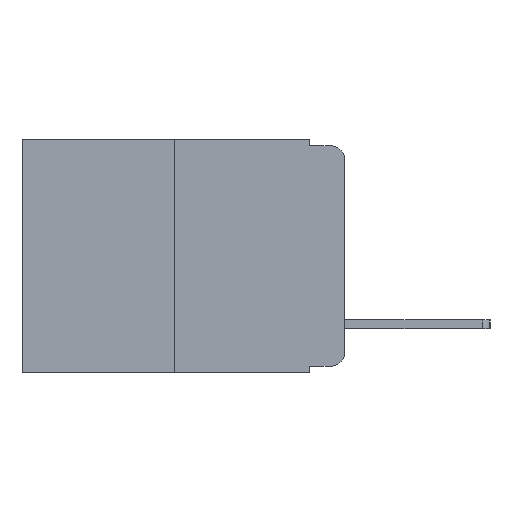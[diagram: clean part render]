
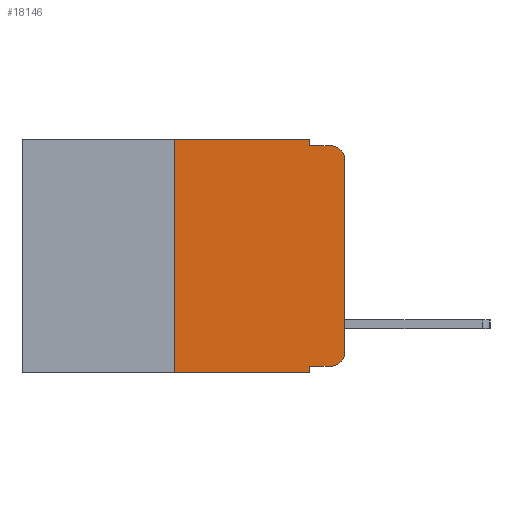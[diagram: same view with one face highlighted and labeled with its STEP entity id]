
A CAD part, left-side view. The second image highlights one B-rep face of the part: STEP entity #18146.
In plain terms, the highlighted planar face has unit normal (-1, 0, 0).
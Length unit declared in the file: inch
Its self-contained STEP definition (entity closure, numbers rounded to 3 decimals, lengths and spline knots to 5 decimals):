
#328 = AXIS2_PLACEMENT_3D ( 'NONE', #8429, #19438, #10042 ) ;
#386 = AXIS2_PLACEMENT_3D ( 'NONE', #10766, #968, #12371 ) ;
#431 = LINE ( 'NONE', #15893, #12927 ) ;
#816 = CIRCLE ( 'NONE', #328, 0.02 ) ;
#943 = EDGE_CURVE ( 'NONE', #11320, #11795, #19920, .T. ) ;
#951 = CARTESIAN_POINT ( 'NONE',  ( 0., 0.02, -0.01 ) ) ;
#968 = DIRECTION ( 'NONE',  ( -1., 0., 0. ) ) ;
#1155 = EDGE_LOOP ( 'NONE', ( #12456, #8713, #17116, #17584, #10220, #2592, #6957, #20031, #3626, #12221 ) ) ;
#1564 = VECTOR ( 'NONE', #10940, 39.37008 ) ;
#2380 = CARTESIAN_POINT ( 'NONE',  ( 0., 0.051, -0.01 ) ) ;
#2413 = VERTEX_POINT ( 'NONE', #951 ) ;
#2592 = ORIENTED_EDGE ( 'NONE', *, *, #20631, .F. ) ;
#2899 = VERTEX_POINT ( 'NONE', #9085 ) ;
#3194 = EDGE_CURVE ( 'NONE', #11320, #19256, #9002, .T. ) ;
#3611 = DIRECTION ( 'NONE',  ( 0., -1., 0. ) ) ;
#3626 = ORIENTED_EDGE ( 'NONE', *, *, #3194, .T. ) ;
#4764 = CARTESIAN_POINT ( 'NONE',  ( 0., 0.051, -0.333 ) ) ;
#4831 = VERTEX_POINT ( 'NONE', #5132 ) ;
#5132 = CARTESIAN_POINT ( 'NONE',  ( 0., 0.051, 0. ) ) ;
#5182 = CARTESIAN_POINT ( 'NONE',  ( 0., 0.02, -0.333 ) ) ;
#5317 = CIRCLE ( 'NONE', #386, 0.02 ) ;
#5368 = PLANE ( 'NONE',  #10641 ) ;
#5703 = VECTOR ( 'NONE', #14656, 39.37008 ) ;
#5969 = LINE ( 'NONE', #15633, #1564 ) ;
#6224 = CARTESIAN_POINT ( 'NONE',  ( 0., 0.051, 0. ) ) ;
#6516 = EDGE_CURVE ( 'NONE', #19256, #17461, #816, .T. ) ;
#6718 = CARTESIAN_POINT ( 'NONE',  ( 0., 0.473, -0.343 ) ) ;
#6886 = CARTESIAN_POINT ( 'NONE',  ( 0., 0., -0.313 ) ) ;
#6957 = ORIENTED_EDGE ( 'NONE', *, *, #19819, .T. ) ;
#6997 = CARTESIAN_POINT ( 'NONE',  ( 0., 0.473, 0. ) ) ;
#7108 = DIRECTION ( 'NONE',  ( 0., 0., -1. ) ) ;
#7861 = VECTOR ( 'NONE', #8493, 39.37008 ) ;
#8353 = LINE ( 'NONE', #13217, #7861 ) ;
#8429 = CARTESIAN_POINT ( 'NONE',  ( 0., 0.02, -0.313 ) ) ;
#8493 = DIRECTION ( 'NONE',  ( 0., -1., 0. ) ) ;
#8618 = DIRECTION ( 'NONE',  ( 1., 0., 0. ) ) ;
#8713 = ORIENTED_EDGE ( 'NONE', *, *, #10140, .T. ) ;
#8808 = CARTESIAN_POINT ( 'NONE',  ( 0., 0.051, -0.333 ) ) ;
#9002 = LINE ( 'NONE', #4764, #13226 ) ;
#9069 = EDGE_CURVE ( 'NONE', #17461, #2899, #10118, .T. ) ;
#9085 = CARTESIAN_POINT ( 'NONE',  ( 0., 0., -0.03 ) ) ;
#9114 = VECTOR ( 'NONE', #18832, 39.37008 ) ;
#9120 = CARTESIAN_POINT ( 'NONE',  ( 0., 0.25, -0.343 ) ) ;
#9368 = EDGE_CURVE ( 'NONE', #16177, #4831, #8353, .T. ) ;
#10042 = DIRECTION ( 'NONE',  ( 0., 0., -1. ) ) ;
#10118 = LINE ( 'NONE', #14135, #9114 ) ;
#10140 = EDGE_CURVE ( 'NONE', #2899, #2413, #5317, .T. ) ;
#10220 = ORIENTED_EDGE ( 'NONE', *, *, #9368, .F. ) ;
#10641 = AXIS2_PLACEMENT_3D ( 'NONE', #6997, #8618, #19609 ) ;
#10766 = CARTESIAN_POINT ( 'NONE',  ( 0., 0.02, -0.03 ) ) ;
#10940 = DIRECTION ( 'NONE',  ( 0., 0., -1. ) ) ;
#11198 = DIRECTION ( 'NONE',  ( 0., 0., 1. ) ) ;
#11320 = VERTEX_POINT ( 'NONE', #8808 ) ;
#11341 = VECTOR ( 'NONE', #3611, 39.37008 ) ;
#11366 = VERTEX_POINT ( 'NONE', #2380 ) ;
#11509 = FACE_OUTER_BOUND ( 'NONE', #1155, .T. ) ;
#11795 = VERTEX_POINT ( 'NONE', #13366 ) ;
#11881 = DIRECTION ( 'NONE',  ( 0., -1., 0. ) ) ;
#12221 = ORIENTED_EDGE ( 'NONE', *, *, #6516, .T. ) ;
#12344 = LINE ( 'NONE', #17905, #11341 ) ;
#12371 = DIRECTION ( 'NONE',  ( 0., 0., -1. ) ) ;
#12456 = ORIENTED_EDGE ( 'NONE', *, *, #9069, .T. ) ;
#12927 = VECTOR ( 'NONE', #11198, 39.37008 ) ;
#13217 = CARTESIAN_POINT ( 'NONE',  ( 0., 0.473, 0. ) ) ;
#13226 = VECTOR ( 'NONE', #11881, 39.37008 ) ;
#13366 = CARTESIAN_POINT ( 'NONE',  ( 0., 0.051, -0.343 ) ) ;
#13980 = CARTESIAN_POINT ( 'NONE',  ( 0., 0.25, 0. ) ) ;
#14135 = CARTESIAN_POINT ( 'NONE',  ( 0., 0., 0. ) ) ;
#14189 = LINE ( 'NONE', #6718, #5703 ) ;
#14656 = DIRECTION ( 'NONE',  ( 0., -1., 0. ) ) ;
#15633 = CARTESIAN_POINT ( 'NONE',  ( 0., 0.051, 0. ) ) ;
#15815 = VECTOR ( 'NONE', #7108, 39.37008 ) ;
#15893 = CARTESIAN_POINT ( 'NONE',  ( 0., 0.25, 0. ) ) ;
#16177 = VERTEX_POINT ( 'NONE', #13980 ) ;
#16487 = EDGE_CURVE ( 'NONE', #11366, #2413, #12344, .T. ) ;
#17116 = ORIENTED_EDGE ( 'NONE', *, *, #16487, .F. ) ;
#17461 = VERTEX_POINT ( 'NONE', #6886 ) ;
#17584 = ORIENTED_EDGE ( 'NONE', *, *, #19589, .F. ) ;
#17905 = CARTESIAN_POINT ( 'NONE',  ( 0., 0.051, -0.01 ) ) ;
#18146 = ADVANCED_FACE ( 'NONE', ( #11509 ), #5368, .F. ) ;
#18832 = DIRECTION ( 'NONE',  ( 0., 0., 1. ) ) ;
#19256 = VERTEX_POINT ( 'NONE', #5182 ) ;
#19438 = DIRECTION ( 'NONE',  ( -1., 0., 0. ) ) ;
#19589 = EDGE_CURVE ( 'NONE', #4831, #11366, #5969, .T. ) ;
#19609 = DIRECTION ( 'NONE',  ( 0., 0., -1. ) ) ;
#19819 = EDGE_CURVE ( 'NONE', #20404, #11795, #14189, .T. ) ;
#19920 = LINE ( 'NONE', #6224, #15815 ) ;
#20031 = ORIENTED_EDGE ( 'NONE', *, *, #943, .F. ) ;
#20404 = VERTEX_POINT ( 'NONE', #9120 ) ;
#20631 = EDGE_CURVE ( 'NONE', #20404, #16177, #431, .T. ) ;
